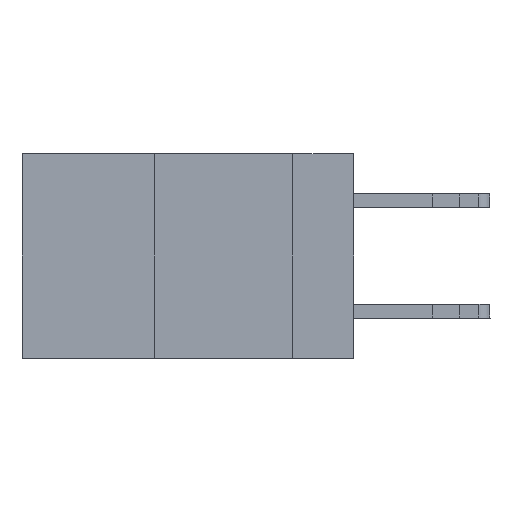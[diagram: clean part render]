
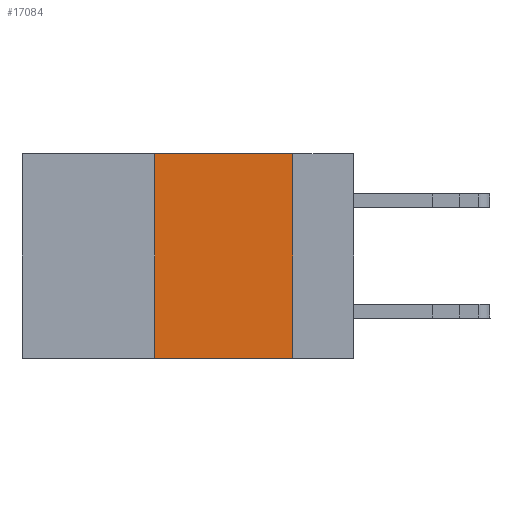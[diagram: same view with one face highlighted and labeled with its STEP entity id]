
A CAD part, left-side view. The second image highlights one B-rep face of the part: STEP entity #17084.
In plain terms, the highlighted planar face has unit normal (-1, 0, 0).
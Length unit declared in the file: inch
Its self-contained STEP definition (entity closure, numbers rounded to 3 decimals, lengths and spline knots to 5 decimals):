
#1755 = DIRECTION ( 'NONE',  ( 0., 0., 1. ) ) ;
#1785 = CARTESIAN_POINT ( 'NONE',  ( 0., 0.36, 0. ) ) ;
#2677 = CARTESIAN_POINT ( 'NONE',  ( 0., 0.11, 0. ) ) ;
#2804 = EDGE_CURVE ( 'NONE', #24244, #25895, #19306, .T. ) ;
#2974 = VECTOR ( 'NONE', #8887, 39.37008 ) ;
#2975 = ORIENTED_EDGE ( 'NONE', *, *, #2804, .T. ) ;
#3768 = DIRECTION ( 'NONE',  ( 0., 0., -1. ) ) ;
#3901 = CARTESIAN_POINT ( 'NONE',  ( 0., 0.36, 0. ) ) ;
#4807 = AXIS2_PLACEMENT_3D ( 'NONE', #14437, #27625, #3768 ) ;
#5464 = CARTESIAN_POINT ( 'NONE',  ( 0., 0.6, 0. ) ) ;
#6007 = DIRECTION ( 'NONE',  ( 0., -1., 0. ) ) ;
#6039 = PLANE ( 'NONE',  #4807 ) ;
#6071 = VECTOR ( 'NONE', #1755, 39.37008 ) ;
#6567 = VECTOR ( 'NONE', #16707, 39.37008 ) ;
#8887 = DIRECTION ( 'NONE',  ( 0., 0., -1. ) ) ;
#9407 = EDGE_LOOP ( 'NONE', ( #21127, #27827, #11226, #2975 ) ) ;
#9864 = EDGE_CURVE ( 'NONE', #19761, #11025, #10862, .T. ) ;
#10443 = CARTESIAN_POINT ( 'NONE',  ( 0., 0.11, -0.37 ) ) ;
#10862 = LINE ( 'NONE', #5464, #17245 ) ;
#11025 = VERTEX_POINT ( 'NONE', #12391 ) ;
#11226 = ORIENTED_EDGE ( 'NONE', *, *, #11769, .F. ) ;
#11769 = EDGE_CURVE ( 'NONE', #24244, #19761, #12414, .T. ) ;
#12372 = LINE ( 'NONE', #2677, #2974 ) ;
#12391 = CARTESIAN_POINT ( 'NONE',  ( 0., 0.11, 0. ) ) ;
#12408 = EDGE_CURVE ( 'NONE', #11025, #25895, #12372, .T. ) ;
#12414 = LINE ( 'NONE', #3901, #6071 ) ;
#14437 = CARTESIAN_POINT ( 'NONE',  ( 0., 0.6, 0. ) ) ;
#16707 = DIRECTION ( 'NONE',  ( 0., -1., 0. ) ) ;
#17084 = ADVANCED_FACE ( 'NONE', ( #27691 ), #6039, .F. ) ;
#17245 = VECTOR ( 'NONE', #6007, 39.37008 ) ;
#17624 = CARTESIAN_POINT ( 'NONE',  ( 0., 0.36, -0.37 ) ) ;
#19306 = LINE ( 'NONE', #20737, #6567 ) ;
#19761 = VERTEX_POINT ( 'NONE', #1785 ) ;
#20737 = CARTESIAN_POINT ( 'NONE',  ( 0., 0.6, -0.37 ) ) ;
#21127 = ORIENTED_EDGE ( 'NONE', *, *, #12408, .F. ) ;
#24244 = VERTEX_POINT ( 'NONE', #17624 ) ;
#25895 = VERTEX_POINT ( 'NONE', #10443 ) ;
#27625 = DIRECTION ( 'NONE',  ( 1., 0., 0. ) ) ;
#27691 = FACE_OUTER_BOUND ( 'NONE', #9407, .T. ) ;
#27827 = ORIENTED_EDGE ( 'NONE', *, *, #9864, .F. ) ;
